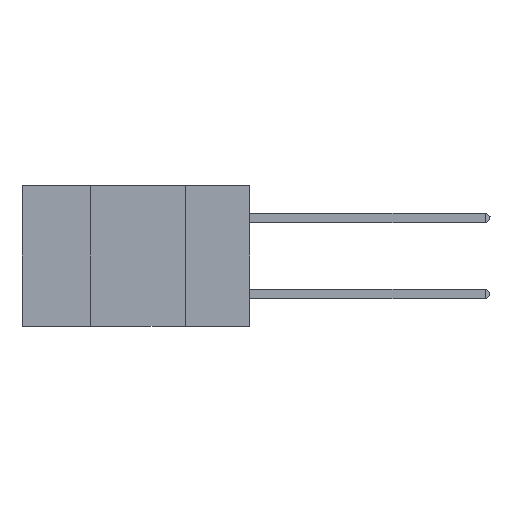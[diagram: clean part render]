
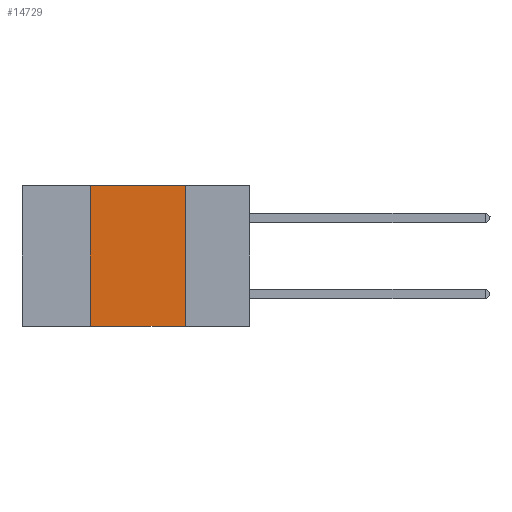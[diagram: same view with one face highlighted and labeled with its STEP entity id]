
A CAD part, left-side view. The second image highlights one B-rep face of the part: STEP entity #14729.
In plain terms, the highlighted planar face has unit normal (-1, 0, 0).
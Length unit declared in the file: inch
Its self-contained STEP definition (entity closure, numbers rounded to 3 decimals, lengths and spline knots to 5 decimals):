
#179 = ORIENTED_EDGE ( 'NONE', *, *, #12008, .F. ) ;
#693 = EDGE_CURVE ( 'NONE', #4673, #12861, #13379, .T. ) ;
#1295 = PLANE ( 'NONE',  #9450 ) ;
#1600 = CARTESIAN_POINT ( 'NONE',  ( 0., 0.17, -0.37 ) ) ;
#2970 = VERTEX_POINT ( 'NONE', #16400 ) ;
#3271 = CARTESIAN_POINT ( 'NONE',  ( 0., 0.6, -0.37 ) ) ;
#3326 = CARTESIAN_POINT ( 'NONE',  ( 0., 0.6, 0. ) ) ;
#3482 = EDGE_CURVE ( 'NONE', #10265, #2970, #14856, .T. ) ;
#4673 = VERTEX_POINT ( 'NONE', #11858 ) ;
#4943 = EDGE_CURVE ( 'NONE', #4673, #10265, #7867, .T. ) ;
#6302 = ORIENTED_EDGE ( 'NONE', *, *, #3482, .F. ) ;
#6418 = CARTESIAN_POINT ( 'NONE',  ( 0., 0.6, 0. ) ) ;
#6508 = DIRECTION ( 'NONE',  ( 0., 0., 1. ) ) ;
#6639 = VECTOR ( 'NONE', #9864, 39.37008 ) ;
#7867 = LINE ( 'NONE', #10228, #12330 ) ;
#8130 = LINE ( 'NONE', #15725, #11936 ) ;
#8380 = ORIENTED_EDGE ( 'NONE', *, *, #693, .T. ) ;
#9450 = AXIS2_PLACEMENT_3D ( 'NONE', #6418, #11572, #10310 ) ;
#9864 = DIRECTION ( 'NONE',  ( 0., -1., 0. ) ) ;
#10228 = CARTESIAN_POINT ( 'NONE',  ( 0., 0.42, 0. ) ) ;
#10265 = VERTEX_POINT ( 'NONE', #16065 ) ;
#10310 = DIRECTION ( 'NONE',  ( 0., 0., -1. ) ) ;
#11572 = DIRECTION ( 'NONE',  ( 1., 0., 0. ) ) ;
#11858 = CARTESIAN_POINT ( 'NONE',  ( 0., 0.42, -0.37 ) ) ;
#11936 = VECTOR ( 'NONE', #14439, 39.37008 ) ;
#12008 = EDGE_CURVE ( 'NONE', #2970, #12861, #8130, .T. ) ;
#12330 = VECTOR ( 'NONE', #6508, 39.37008 ) ;
#12824 = FACE_OUTER_BOUND ( 'NONE', #15712, .T. ) ;
#12861 = VERTEX_POINT ( 'NONE', #1600 ) ;
#13200 = VECTOR ( 'NONE', #13600, 39.37008 ) ;
#13379 = LINE ( 'NONE', #3271, #6639 ) ;
#13600 = DIRECTION ( 'NONE',  ( 0., -1., 0. ) ) ;
#14439 = DIRECTION ( 'NONE',  ( 0., 0., -1. ) ) ;
#14729 = ADVANCED_FACE ( 'NONE', ( #12824 ), #1295, .F. ) ;
#14856 = LINE ( 'NONE', #3326, #13200 ) ;
#15688 = ORIENTED_EDGE ( 'NONE', *, *, #4943, .F. ) ;
#15712 = EDGE_LOOP ( 'NONE', ( #179, #6302, #15688, #8380 ) ) ;
#15725 = CARTESIAN_POINT ( 'NONE',  ( 0., 0.17, 0. ) ) ;
#16065 = CARTESIAN_POINT ( 'NONE',  ( 0., 0.42, 0. ) ) ;
#16400 = CARTESIAN_POINT ( 'NONE',  ( 0., 0.17, 0. ) ) ;
